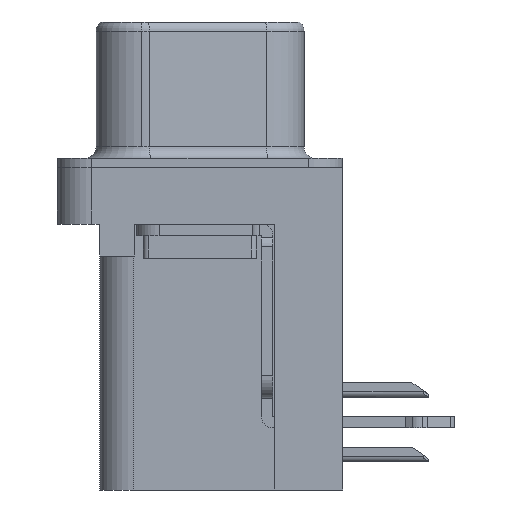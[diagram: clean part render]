
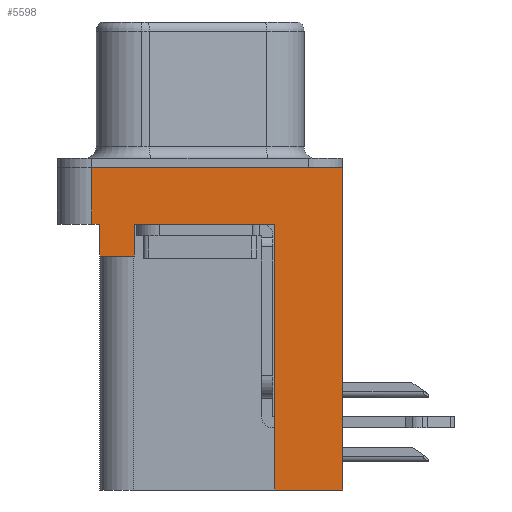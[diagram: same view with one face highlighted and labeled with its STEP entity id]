
A CAD part, left-side view. The second image highlights one B-rep face of the part: STEP entity #5598.
In plain terms, the highlighted planar face has unit normal (-1, 0, 0).
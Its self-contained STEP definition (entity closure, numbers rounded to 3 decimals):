
#88 = ORIENTED_EDGE ( 'NONE', *, *, #6336, .F. ) ;
#233 = EDGE_CURVE ( 'NONE', #14991, #1513, #14949, .T. ) ;
#306 = CARTESIAN_POINT ( 'NONE',  ( -2.935, -3.295, -14.2 ) ) ;
#507 = CARTESIAN_POINT ( 'NONE',  ( -2.935, 4.775, -2.5 ) ) ;
#620 = VECTOR ( 'NONE', #13006, 1000. ) ;
#665 = CARTESIAN_POINT ( 'NONE',  ( -2.935, -3.295, -14.2 ) ) ;
#821 = CARTESIAN_POINT ( 'NONE',  ( -2.935, -6.275, -2.5 ) ) ;
#896 = VECTOR ( 'NONE', #1935, 1000. ) ;
#907 = LINE ( 'NONE', #5170, #620 ) ;
#1018 = EDGE_CURVE ( 'NONE', #14991, #19112, #8955, .T. ) ;
#1024 = PLANE ( 'NONE',  #3675 ) ;
#1199 = CARTESIAN_POINT ( 'NONE',  ( -2.935, -6.275, 0. ) ) ;
#1222 = CARTESIAN_POINT ( 'NONE',  ( -2.935, -3.295, -2.5 ) ) ;
#1256 = DIRECTION ( 'NONE',  ( 0., 1., 0. ) ) ;
#1269 = LINE ( 'NONE', #18321, #10722 ) ;
#1428 = ORIENTED_EDGE ( 'NONE', *, *, #13707, .F. ) ;
#1508 = LINE ( 'NONE', #8940, #13902 ) ;
#1513 = VERTEX_POINT ( 'NONE', #14953 ) ;
#1898 = VECTOR ( 'NONE', #11752, 1000. ) ;
#1935 = DIRECTION ( 'NONE',  ( 0., 0., 1. ) ) ;
#2093 = VECTOR ( 'NONE', #2782, 1000. ) ;
#2403 = VERTEX_POINT ( 'NONE', #13721 ) ;
#2586 = EDGE_CURVE ( 'NONE', #12264, #2403, #12622, .T. ) ;
#2611 = DIRECTION ( 'NONE',  ( -1., 0., 0. ) ) ;
#2695 = VECTOR ( 'NONE', #5178, 1000. ) ;
#2769 = VERTEX_POINT ( 'NONE', #5480 ) ;
#2782 = DIRECTION ( 'NONE',  ( 0., -1., 0. ) ) ;
#3590 = EDGE_CURVE ( 'NONE', #19112, #5632, #12748, .T. ) ;
#3675 = AXIS2_PLACEMENT_3D ( 'NONE', #821, #2611, #13116 ) ;
#3721 = VECTOR ( 'NONE', #1256, 1000. ) ;
#4890 = LINE ( 'NONE', #10950, #9068 ) ;
#4950 = ORIENTED_EDGE ( 'NONE', *, *, #2586, .F. ) ;
#5170 = CARTESIAN_POINT ( 'NONE',  ( -2.935, -6.275, -2.5 ) ) ;
#5178 = DIRECTION ( 'NONE',  ( 0., 0., 1. ) ) ;
#5480 = CARTESIAN_POINT ( 'NONE',  ( -2.935, 2.895, -2.5 ) ) ;
#5598 = ADVANCED_FACE ( 'NONE', ( #9856 ), #1024, .T. ) ;
#5632 = VERTEX_POINT ( 'NONE', #1222 ) ;
#6336 = EDGE_CURVE ( 'NONE', #10548, #1513, #7331, .T. ) ;
#6462 = CARTESIAN_POINT ( 'NONE',  ( -2.935, 4.425, -3.9 ) ) ;
#7233 = ORIENTED_EDGE ( 'NONE', *, *, #9114, .F. ) ;
#7331 = LINE ( 'NONE', #1199, #2093 ) ;
#7508 = CARTESIAN_POINT ( 'NONE',  ( -2.935, -6.275, -2.5 ) ) ;
#8215 = CARTESIAN_POINT ( 'NONE',  ( -2.935, -6.275, -14.2 ) ) ;
#8265 = CARTESIAN_POINT ( 'NONE',  ( -2.935, 2.895, -3.9 ) ) ;
#8389 = VERTEX_POINT ( 'NONE', #507 ) ;
#8940 = CARTESIAN_POINT ( 'NONE',  ( -2.935, 2.895, -3.9 ) ) ;
#8955 = LINE ( 'NONE', #306, #1898 ) ;
#9068 = VECTOR ( 'NONE', #18691, 1000. ) ;
#9114 = EDGE_CURVE ( 'NONE', #8389, #10548, #1269, .T. ) ;
#9416 = ORIENTED_EDGE ( 'NONE', *, *, #14620, .T. ) ;
#9460 = EDGE_LOOP ( 'NONE', ( #88, #7233, #9416, #4950, #1428, #15266, #10028, #11374, #10904, #17797 ) ) ;
#9856 = FACE_OUTER_BOUND ( 'NONE', #9460, .T. ) ;
#10028 = ORIENTED_EDGE ( 'NONE', *, *, #11047, .T. ) ;
#10050 = EDGE_CURVE ( 'NONE', #18516, #2769, #1508, .T. ) ;
#10548 = VERTEX_POINT ( 'NONE', #11078 ) ;
#10722 = VECTOR ( 'NONE', #12364, 1000. ) ;
#10802 = VECTOR ( 'NONE', #13855, 1000. ) ;
#10904 = ORIENTED_EDGE ( 'NONE', *, *, #1018, .F. ) ;
#10950 = CARTESIAN_POINT ( 'NONE',  ( -2.935, -6.275, -2.5 ) ) ;
#11047 = EDGE_CURVE ( 'NONE', #2769, #5632, #4890, .T. ) ;
#11078 = CARTESIAN_POINT ( 'NONE',  ( -2.935, 4.775, 0. ) ) ;
#11251 = CARTESIAN_POINT ( 'NONE',  ( -2.935, 4.425, -3.9 ) ) ;
#11374 = ORIENTED_EDGE ( 'NONE', *, *, #3590, .F. ) ;
#11752 = DIRECTION ( 'NONE',  ( 0., 1., 0. ) ) ;
#12264 = VERTEX_POINT ( 'NONE', #11251 ) ;
#12364 = DIRECTION ( 'NONE',  ( 0., 0., 1. ) ) ;
#12622 = LINE ( 'NONE', #6462, #2695 ) ;
#12748 = LINE ( 'NONE', #15611, #896 ) ;
#13006 = DIRECTION ( 'NONE',  ( 0., -1., 0. ) ) ;
#13116 = DIRECTION ( 'NONE',  ( 0., 0., 1. ) ) ;
#13707 = EDGE_CURVE ( 'NONE', #18516, #12264, #19514, .T. ) ;
#13721 = CARTESIAN_POINT ( 'NONE',  ( -2.935, 4.425, -2.5 ) ) ;
#13855 = DIRECTION ( 'NONE',  ( 0., 0., 1. ) ) ;
#13902 = VECTOR ( 'NONE', #15082, 1000. ) ;
#14620 = EDGE_CURVE ( 'NONE', #8389, #2403, #907, .T. ) ;
#14925 = CARTESIAN_POINT ( 'NONE',  ( -2.935, 4.425, -3.9 ) ) ;
#14949 = LINE ( 'NONE', #7508, #10802 ) ;
#14953 = CARTESIAN_POINT ( 'NONE',  ( -2.935, -6.275, 0. ) ) ;
#14991 = VERTEX_POINT ( 'NONE', #8215 ) ;
#15082 = DIRECTION ( 'NONE',  ( 0., 0., 1. ) ) ;
#15266 = ORIENTED_EDGE ( 'NONE', *, *, #10050, .T. ) ;
#15611 = CARTESIAN_POINT ( 'NONE',  ( -2.935, -3.295, -14.2 ) ) ;
#17797 = ORIENTED_EDGE ( 'NONE', *, *, #233, .T. ) ;
#18321 = CARTESIAN_POINT ( 'NONE',  ( -2.935, 4.775, -2.5 ) ) ;
#18516 = VERTEX_POINT ( 'NONE', #8265 ) ;
#18691 = DIRECTION ( 'NONE',  ( 0., -1., 0. ) ) ;
#19112 = VERTEX_POINT ( 'NONE', #665 ) ;
#19514 = LINE ( 'NONE', #14925, #3721 ) ;
